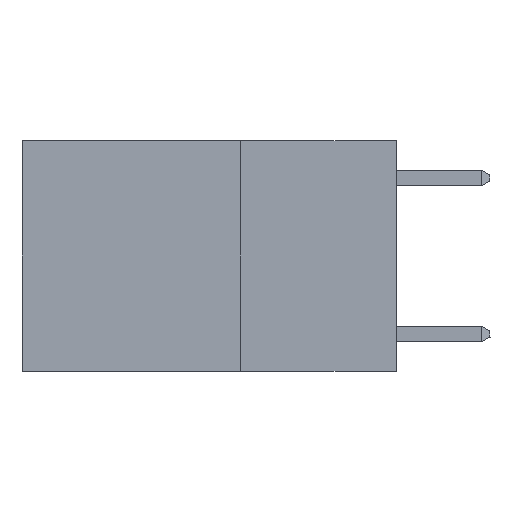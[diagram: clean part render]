
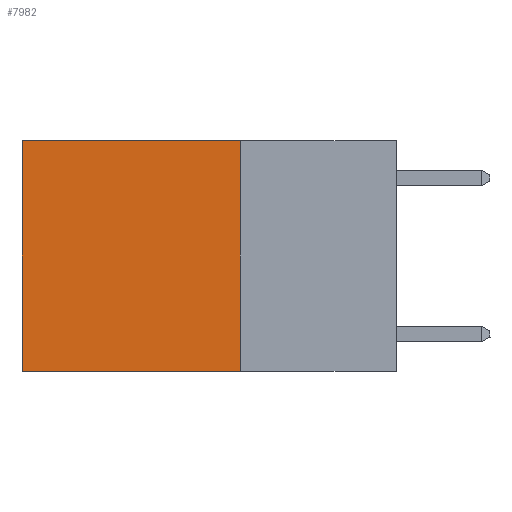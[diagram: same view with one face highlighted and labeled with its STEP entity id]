
A CAD part, left-side view. The second image highlights one B-rep face of the part: STEP entity #7982.
In plain terms, the highlighted planar face has unit normal (-1, 0, 0).
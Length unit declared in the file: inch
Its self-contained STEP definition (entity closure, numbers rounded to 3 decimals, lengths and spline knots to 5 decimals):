
#417 = EDGE_LOOP ( 'NONE', ( #12434, #5546, #12038, #10173 ) ) ;
#811 = LINE ( 'NONE', #11271, #9171 ) ;
#972 = CARTESIAN_POINT ( 'NONE',  ( 0.2625, 0.25, -0.37 ) ) ;
#1916 = AXIS2_PLACEMENT_3D ( 'NONE', #10219, #3924, #11276 ) ;
#2862 = EDGE_CURVE ( 'NONE', #10355, #4641, #4248, .T. ) ;
#3780 = DIRECTION ( 'NONE',  ( 0., 1., 0. ) ) ;
#3924 = DIRECTION ( 'NONE',  ( 1., 0., 0. ) ) ;
#4248 = LINE ( 'NONE', #972, #6698 ) ;
#4641 = VERTEX_POINT ( 'NONE', #9377 ) ;
#4913 = LINE ( 'NONE', #11134, #7049 ) ;
#4957 = DIRECTION ( 'NONE',  ( 0., 0., -1. ) ) ;
#5465 = VERTEX_POINT ( 'NONE', #12827 ) ;
#5546 = ORIENTED_EDGE ( 'NONE', *, *, #2862, .F. ) ;
#6698 = VECTOR ( 'NONE', #8308, 39.37008 ) ;
#7049 = VECTOR ( 'NONE', #3780, 39.37008 ) ;
#7135 = VECTOR ( 'NONE', #9614, 39.37008 ) ;
#7982 = ADVANCED_FACE ( 'NONE', ( #8801 ), #9081, .F. ) ;
#8308 = DIRECTION ( 'NONE',  ( 0., 1., 0. ) ) ;
#8541 = CARTESIAN_POINT ( 'NONE',  ( 0.2625, 0.25, 0. ) ) ;
#8796 = CARTESIAN_POINT ( 'NONE',  ( 0.2625, 0.25, -0.37 ) ) ;
#8801 = FACE_OUTER_BOUND ( 'NONE', #417, .T. ) ;
#9081 = PLANE ( 'NONE',  #1916 ) ;
#9171 = VECTOR ( 'NONE', #4957, 39.37008 ) ;
#9377 = CARTESIAN_POINT ( 'NONE',  ( 0.2625, 0.6, -0.37 ) ) ;
#9508 = EDGE_CURVE ( 'NONE', #5465, #10355, #13406, .T. ) ;
#9614 = DIRECTION ( 'NONE',  ( 0., 0., -1. ) ) ;
#9884 = VERTEX_POINT ( 'NONE', #10129 ) ;
#10129 = CARTESIAN_POINT ( 'NONE',  ( 0.2625, 0.6, 0. ) ) ;
#10173 = ORIENTED_EDGE ( 'NONE', *, *, #13004, .T. ) ;
#10219 = CARTESIAN_POINT ( 'NONE',  ( 0.2625, 0.25, 0. ) ) ;
#10355 = VERTEX_POINT ( 'NONE', #8796 ) ;
#11134 = CARTESIAN_POINT ( 'NONE',  ( 0.2625, 0.25, 0. ) ) ;
#11271 = CARTESIAN_POINT ( 'NONE',  ( 0.2625, 0.6, 0. ) ) ;
#11276 = DIRECTION ( 'NONE',  ( 0., 0., -1. ) ) ;
#12038 = ORIENTED_EDGE ( 'NONE', *, *, #9508, .F. ) ;
#12434 = ORIENTED_EDGE ( 'NONE', *, *, #13073, .T. ) ;
#12827 = CARTESIAN_POINT ( 'NONE',  ( 0.2625, 0.25, 0. ) ) ;
#13004 = EDGE_CURVE ( 'NONE', #5465, #9884, #4913, .T. ) ;
#13073 = EDGE_CURVE ( 'NONE', #9884, #4641, #811, .T. ) ;
#13406 = LINE ( 'NONE', #8541, #7135 ) ;
